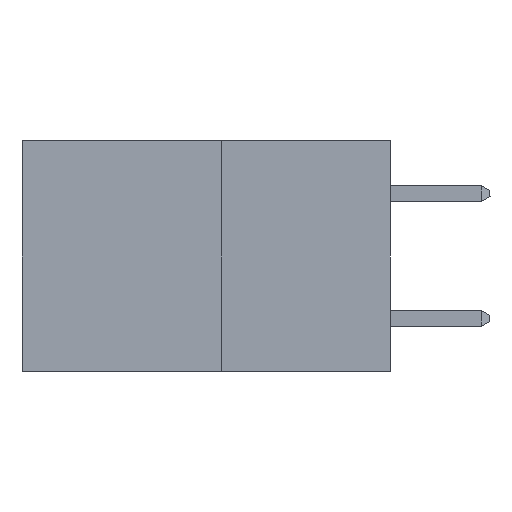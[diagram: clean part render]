
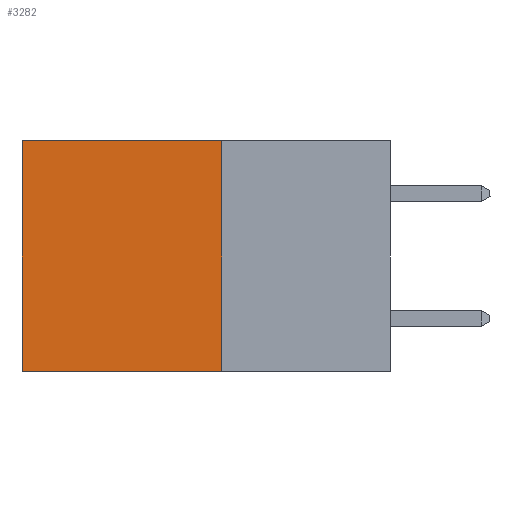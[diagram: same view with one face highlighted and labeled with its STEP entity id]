
A CAD part, left-side view. The second image highlights one B-rep face of the part: STEP entity #3282.
In plain terms, the highlighted planar face has unit normal (-1, 0, 0).
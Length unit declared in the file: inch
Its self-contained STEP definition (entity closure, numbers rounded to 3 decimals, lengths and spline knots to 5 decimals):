
#274 = LINE ( 'NONE', #5646, #5485 ) ;
#1681 = CARTESIAN_POINT ( 'NONE',  ( 0.277, 0.27, 0. ) ) ;
#2484 = CARTESIAN_POINT ( 'NONE',  ( 0.277, 0.27, -0.37 ) ) ;
#3270 = LINE ( 'NONE', #1681, #12990 ) ;
#3282 = ADVANCED_FACE ( 'NONE', ( #5989 ), #22427, .F. ) ;
#3479 = ORIENTED_EDGE ( 'NONE', *, *, #16317, .T. ) ;
#3482 = VECTOR ( 'NONE', #8921, 39.37008 ) ;
#4321 = EDGE_CURVE ( 'NONE', #15886, #22710, #13203, .T. ) ;
#5485 = VECTOR ( 'NONE', #19255, 39.37008 ) ;
#5540 = ORIENTED_EDGE ( 'NONE', *, *, #4321, .F. ) ;
#5646 = CARTESIAN_POINT ( 'NONE',  ( 0.277, 0.59, -0.37 ) ) ;
#5989 = FACE_OUTER_BOUND ( 'NONE', #12595, .T. ) ;
#7593 = AXIS2_PLACEMENT_3D ( 'NONE', #19499, #18468, #18269 ) ;
#8014 = CARTESIAN_POINT ( 'NONE',  ( 0.277, 0.27, -0.37 ) ) ;
#8863 = CARTESIAN_POINT ( 'NONE',  ( 0.277, 0.59, -0.37 ) ) ;
#8921 = DIRECTION ( 'NONE',  ( 0., 1., 0. ) ) ;
#9671 = CARTESIAN_POINT ( 'NONE',  ( 0.277, 0.27, -0.37 ) ) ;
#12595 = EDGE_LOOP ( 'NONE', ( #3479, #5540, #15130, #20009 ) ) ;
#12990 = VECTOR ( 'NONE', #24783, 39.37008 ) ;
#13203 = LINE ( 'NONE', #8014, #3482 ) ;
#14593 = LINE ( 'NONE', #9671, #24170 ) ;
#15130 = ORIENTED_EDGE ( 'NONE', *, *, #16397, .F. ) ;
#15886 = VERTEX_POINT ( 'NONE', #2484 ) ;
#16317 = EDGE_CURVE ( 'NONE', #20636, #22710, #274, .T. ) ;
#16397 = EDGE_CURVE ( 'NONE', #17498, #15886, #14593, .T. ) ;
#17498 = VERTEX_POINT ( 'NONE', #24048 ) ;
#18269 = DIRECTION ( 'NONE',  ( 0., 0., -1. ) ) ;
#18468 = DIRECTION ( 'NONE',  ( 1., 0., 0. ) ) ;
#18708 = CARTESIAN_POINT ( 'NONE',  ( 0.277, 0.59, 0. ) ) ;
#19255 = DIRECTION ( 'NONE',  ( 0., 0., -1. ) ) ;
#19499 = CARTESIAN_POINT ( 'NONE',  ( 0.277, 0.27, -0.37 ) ) ;
#20009 = ORIENTED_EDGE ( 'NONE', *, *, #24154, .T. ) ;
#20636 = VERTEX_POINT ( 'NONE', #18708 ) ;
#22427 = PLANE ( 'NONE',  #7593 ) ;
#22710 = VERTEX_POINT ( 'NONE', #8863 ) ;
#24048 = CARTESIAN_POINT ( 'NONE',  ( 0.277, 0.27, 0. ) ) ;
#24154 = EDGE_CURVE ( 'NONE', #17498, #20636, #3270, .T. ) ;
#24170 = VECTOR ( 'NONE', #24980, 39.37008 ) ;
#24783 = DIRECTION ( 'NONE',  ( 0., 1., 0. ) ) ;
#24980 = DIRECTION ( 'NONE',  ( 0., 0., -1. ) ) ;
